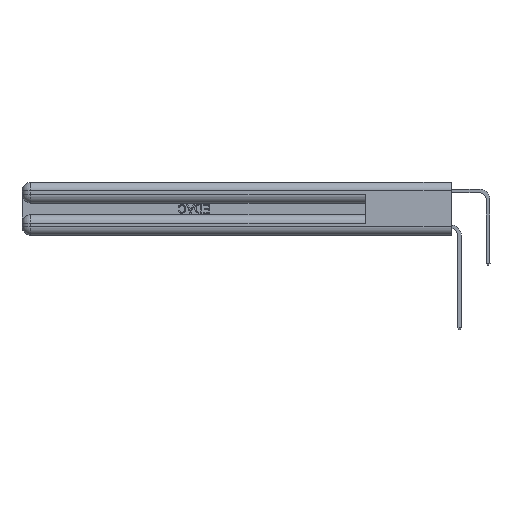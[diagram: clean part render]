
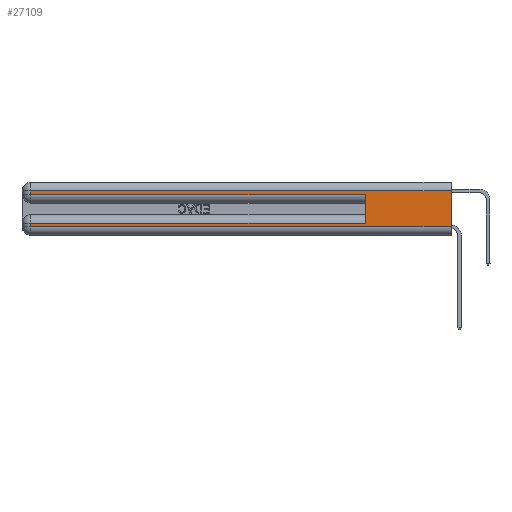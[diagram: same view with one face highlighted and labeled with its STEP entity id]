
A CAD part, left-side view. The second image highlights one B-rep face of the part: STEP entity #27109.
In plain terms, the highlighted planar face has unit normal (-1, 0, 0).
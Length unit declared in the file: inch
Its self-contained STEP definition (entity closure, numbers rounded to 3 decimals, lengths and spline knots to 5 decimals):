
#1175 = DIRECTION ( 'NONE',  ( 0., 0., -1. ) ) ;
#1519 = CARTESIAN_POINT ( 'NONE',  ( 0., 0., 0.31 ) ) ;
#1959 = ORIENTED_EDGE ( 'NONE', *, *, #10261, .T. ) ;
#2252 = ORIENTED_EDGE ( 'NONE', *, *, #14228, .T. ) ;
#2262 = CARTESIAN_POINT ( 'NONE',  ( 0., 0., 0.06 ) ) ;
#2357 = DIRECTION ( 'NONE',  ( 0., 0., 1. ) ) ;
#2590 = CARTESIAN_POINT ( 'NONE',  ( 0., 0.6, 0.285 ) ) ;
#2630 = LINE ( 'NONE', #13909, #17828 ) ;
#3004 = VERTEX_POINT ( 'NONE', #13776 ) ;
#3345 = CARTESIAN_POINT ( 'NONE',  ( 0., 2.94, 0.085 ) ) ;
#3583 = FACE_OUTER_BOUND ( 'NONE', #16042, .T. ) ;
#3740 = DIRECTION ( 'NONE',  ( 1., 0., 0. ) ) ;
#4670 = ORIENTED_EDGE ( 'NONE', *, *, #25426, .T. ) ;
#5907 = CARTESIAN_POINT ( 'NONE',  ( 0., 0., 0.37 ) ) ;
#6647 = CARTESIAN_POINT ( 'NONE',  ( 0., 0., 0.085 ) ) ;
#7012 = DIRECTION ( 'NONE',  ( 0., -1., 0. ) ) ;
#7869 = EDGE_CURVE ( 'NONE', #18296, #19296, #13190, .T. ) ;
#8163 = ORIENTED_EDGE ( 'NONE', *, *, #21536, .F. ) ;
#8210 = EDGE_CURVE ( 'NONE', #19574, #23289, #20179, .T. ) ;
#8749 = DIRECTION ( 'NONE',  ( 0., 1., 0. ) ) ;
#8890 = CARTESIAN_POINT ( 'NONE',  ( 0., 0., 0.285 ) ) ;
#10261 = EDGE_CURVE ( 'NONE', #3004, #24530, #25290, .T. ) ;
#10893 = DIRECTION ( 'NONE',  ( 0., 0., -1. ) ) ;
#11816 = VERTEX_POINT ( 'NONE', #16919 ) ;
#11863 = VECTOR ( 'NONE', #11957, 39.37008 ) ;
#11957 = DIRECTION ( 'NONE',  ( 0., 0., -1. ) ) ;
#12951 = VECTOR ( 'NONE', #8749, 39.37008 ) ;
#13190 = LINE ( 'NONE', #6647, #21667 ) ;
#13451 = DIRECTION ( 'NONE',  ( 0., -1., 0. ) ) ;
#13776 = CARTESIAN_POINT ( 'NONE',  ( 0., 2.94, 0.06 ) ) ;
#13909 = CARTESIAN_POINT ( 'NONE',  ( 0., 0., 0.37 ) ) ;
#14228 = EDGE_CURVE ( 'NONE', #23289, #11816, #16818, .T. ) ;
#14937 = ORIENTED_EDGE ( 'NONE', *, *, #7869, .T. ) ;
#16042 = EDGE_LOOP ( 'NONE', ( #23824, #16716, #2252, #26724, #8163, #14937, #4670, #1959 ) ) ;
#16343 = VECTOR ( 'NONE', #7012, 39.37008 ) ;
#16716 = ORIENTED_EDGE ( 'NONE', *, *, #8210, .T. ) ;
#16818 = LINE ( 'NONE', #25985, #11863 ) ;
#16919 = CARTESIAN_POINT ( 'NONE',  ( 0., 2.94, 0.285 ) ) ;
#17121 = EDGE_CURVE ( 'NONE', #11816, #23629, #22155, .T. ) ;
#17336 = CARTESIAN_POINT ( 'NONE',  ( 0., 2.94, 0.37 ) ) ;
#17828 = VECTOR ( 'NONE', #21084, 39.37008 ) ;
#18296 = VERTEX_POINT ( 'NONE', #27579 ) ;
#19296 = VERTEX_POINT ( 'NONE', #3345 ) ;
#19574 = VERTEX_POINT ( 'NONE', #1519 ) ;
#19612 = VECTOR ( 'NONE', #13451, 39.37008 ) ;
#20179 = LINE ( 'NONE', #29664, #12951 ) ;
#20199 = DIRECTION ( 'NONE',  ( 0., 1., 0. ) ) ;
#21084 = DIRECTION ( 'NONE',  ( 0., 0., -1. ) ) ;
#21536 = EDGE_CURVE ( 'NONE', #18296, #23629, #25534, .T. ) ;
#21667 = VECTOR ( 'NONE', #20199, 39.37008 ) ;
#22155 = LINE ( 'NONE', #8890, #19612 ) ;
#23212 = VECTOR ( 'NONE', #1175, 39.37008 ) ;
#23226 = CARTESIAN_POINT ( 'NONE',  ( 0., 0.6, 0.145 ) ) ;
#23289 = VERTEX_POINT ( 'NONE', #24106 ) ;
#23629 = VERTEX_POINT ( 'NONE', #2590 ) ;
#23824 = ORIENTED_EDGE ( 'NONE', *, *, #24688, .F. ) ;
#24106 = CARTESIAN_POINT ( 'NONE',  ( 0., 2.94, 0.31 ) ) ;
#24530 = VERTEX_POINT ( 'NONE', #27514 ) ;
#24688 = EDGE_CURVE ( 'NONE', #19574, #24530, #2630, .T. ) ;
#25290 = LINE ( 'NONE', #2262, #16343 ) ;
#25426 = EDGE_CURVE ( 'NONE', #19296, #3004, #29112, .T. ) ;
#25534 = LINE ( 'NONE', #23226, #26076 ) ;
#25743 = AXIS2_PLACEMENT_3D ( 'NONE', #5907, #3740, #10893 ) ;
#25985 = CARTESIAN_POINT ( 'NONE',  ( 0., 2.94, 0.37 ) ) ;
#26076 = VECTOR ( 'NONE', #2357, 39.37008 ) ;
#26472 = PLANE ( 'NONE',  #25743 ) ;
#26724 = ORIENTED_EDGE ( 'NONE', *, *, #17121, .T. ) ;
#27109 = ADVANCED_FACE ( 'NONE', ( #3583 ), #26472, .F. ) ;
#27514 = CARTESIAN_POINT ( 'NONE',  ( 0., 0., 0.06 ) ) ;
#27579 = CARTESIAN_POINT ( 'NONE',  ( 0., 0.6, 0.085 ) ) ;
#29112 = LINE ( 'NONE', #17336, #23212 ) ;
#29664 = CARTESIAN_POINT ( 'NONE',  ( 0., 0., 0.31 ) ) ;
